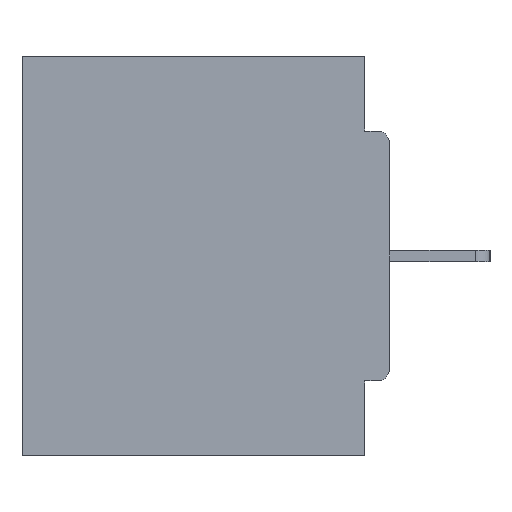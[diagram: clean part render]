
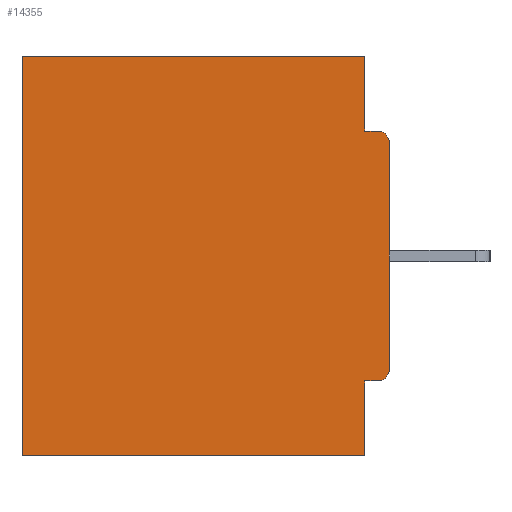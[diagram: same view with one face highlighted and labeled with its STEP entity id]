
A CAD part, left-side view. The second image highlights one B-rep face of the part: STEP entity #14355.
In plain terms, the highlighted planar face has unit normal (-1, 0, 0).
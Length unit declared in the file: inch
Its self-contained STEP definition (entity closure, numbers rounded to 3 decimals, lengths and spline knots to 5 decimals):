
#38 = CARTESIAN_POINT ( 'NONE',  ( 0.298, 0., -0.4065 ) ) ;
#102 = ORIENTED_EDGE ( 'NONE', *, *, #11221, .T. ) ;
#595 = DIRECTION ( 'NONE',  ( -1., 0., 0. ) ) ;
#1660 = LINE ( 'NONE', #21079, #13743 ) ;
#1907 = VERTEX_POINT ( 'NONE', #7659 ) ;
#2743 = CARTESIAN_POINT ( 'NONE',  ( 0.298, 0.015, -0.1085 ) ) ;
#3783 = ORIENTED_EDGE ( 'NONE', *, *, #19556, .F. ) ;
#4271 = EDGE_CURVE ( 'NONE', #1907, #17681, #12947, .T. ) ;
#4318 = CARTESIAN_POINT ( 'NONE',  ( 0.298, 0.031, -0.4065 ) ) ;
#4432 = ORIENTED_EDGE ( 'NONE', *, *, #5031, .F. ) ;
#4503 = DIRECTION ( 'NONE',  ( 1., 0., 0. ) ) ;
#4578 = EDGE_CURVE ( 'NONE', #23569, #7492, #11130, .T. ) ;
#4992 = DIRECTION ( 'NONE',  ( 0., 0., -1. ) ) ;
#5031 = EDGE_CURVE ( 'NONE', #18633, #25274, #25916, .T. ) ;
#5230 = DIRECTION ( 'NONE',  ( 0., 0., -1. ) ) ;
#5578 = VECTOR ( 'NONE', #26715, 39.37008 ) ;
#6106 = DIRECTION ( 'NONE',  ( 0., -1., 0. ) ) ;
#6432 = AXIS2_PLACEMENT_3D ( 'NONE', #2743, #595, #9349 ) ;
#6659 = CARTESIAN_POINT ( 'NONE',  ( 0.298, 0., 0. ) ) ;
#6816 = CARTESIAN_POINT ( 'NONE',  ( 0.298, 0.031, -0.5 ) ) ;
#7492 = VERTEX_POINT ( 'NONE', #19065 ) ;
#7659 = CARTESIAN_POINT ( 'NONE',  ( 0.298, 0.031, 0. ) ) ;
#7872 = CARTESIAN_POINT ( 'NONE',  ( 0.298, 0.015, -0.0935 ) ) ;
#8665 = VERTEX_POINT ( 'NONE', #9202 ) ;
#8872 = DIRECTION ( 'NONE',  ( -1., 0., 0. ) ) ;
#9202 = CARTESIAN_POINT ( 'NONE',  ( 0.298, 0., -0.3915 ) ) ;
#9349 = DIRECTION ( 'NONE',  ( 0., 0., -1. ) ) ;
#9413 = ORIENTED_EDGE ( 'NONE', *, *, #13356, .T. ) ;
#9640 = CIRCLE ( 'NONE', #6432, 0.015 ) ;
#10144 = ORIENTED_EDGE ( 'NONE', *, *, #26848, .T. ) ;
#10217 = LINE ( 'NONE', #12099, #11525 ) ;
#10304 = VECTOR ( 'NONE', #21458, 39.37008 ) ;
#10714 = ORIENTED_EDGE ( 'NONE', *, *, #10889, .F. ) ;
#10738 = ORIENTED_EDGE ( 'NONE', *, *, #12659, .F. ) ;
#10889 = EDGE_CURVE ( 'NONE', #17681, #24503, #1660, .T. ) ;
#11065 = CIRCLE ( 'NONE', #27132, 0.015 ) ;
#11130 = LINE ( 'NONE', #26096, #18118 ) ;
#11221 = EDGE_CURVE ( 'NONE', #17450, #7492, #14136, .T. ) ;
#11470 = CARTESIAN_POINT ( 'NONE',  ( 0.298, 0., -0.1085 ) ) ;
#11479 = CARTESIAN_POINT ( 'NONE',  ( 0.298, 0., 0. ) ) ;
#11525 = VECTOR ( 'NONE', #24638, 39.37008 ) ;
#11661 = EDGE_CURVE ( 'NONE', #12113, #24503, #9640, .T. ) ;
#12099 = CARTESIAN_POINT ( 'NONE',  ( 0.298, 0.031, -0.5 ) ) ;
#12113 = VERTEX_POINT ( 'NONE', #11470 ) ;
#12446 = AXIS2_PLACEMENT_3D ( 'NONE', #6659, #4503, #13289 ) ;
#12659 = EDGE_CURVE ( 'NONE', #25274, #23569, #10217, .T. ) ;
#12947 = LINE ( 'NONE', #19554, #15370 ) ;
#13289 = DIRECTION ( 'NONE',  ( 0., 0., -1. ) ) ;
#13356 = EDGE_CURVE ( 'NONE', #1907, #17450, #13492, .T. ) ;
#13492 = LINE ( 'NONE', #11479, #5578 ) ;
#13743 = VECTOR ( 'NONE', #6106, 39.37008 ) ;
#14115 = LINE ( 'NONE', #16570, #14943 ) ;
#14136 = LINE ( 'NONE', #20199, #18360 ) ;
#14355 = ADVANCED_FACE ( 'NONE', ( #17603 ), #24481, .F. ) ;
#14943 = VECTOR ( 'NONE', #23179, 39.37008 ) ;
#15370 = VECTOR ( 'NONE', #19130, 39.37008 ) ;
#16570 = CARTESIAN_POINT ( 'NONE',  ( 0.298, 0., 0. ) ) ;
#17450 = VERTEX_POINT ( 'NONE', #18506 ) ;
#17603 = FACE_OUTER_BOUND ( 'NONE', #24898, .T. ) ;
#17681 = VERTEX_POINT ( 'NONE', #23815 ) ;
#18078 = CARTESIAN_POINT ( 'NONE',  ( 0.298, 0.015, -0.3915 ) ) ;
#18118 = VECTOR ( 'NONE', #19628, 39.37008 ) ;
#18360 = VECTOR ( 'NONE', #5230, 39.37008 ) ;
#18506 = CARTESIAN_POINT ( 'NONE',  ( 0.298, 0.46, 0. ) ) ;
#18633 = VERTEX_POINT ( 'NONE', #22580 ) ;
#18969 = ORIENTED_EDGE ( 'NONE', *, *, #4271, .F. ) ;
#19065 = CARTESIAN_POINT ( 'NONE',  ( 0.298, 0.46, -0.5 ) ) ;
#19130 = DIRECTION ( 'NONE',  ( 0., 0., -1. ) ) ;
#19554 = CARTESIAN_POINT ( 'NONE',  ( 0.298, 0.031, -0.5 ) ) ;
#19556 = EDGE_CURVE ( 'NONE', #12113, #8665, #14115, .T. ) ;
#19628 = DIRECTION ( 'NONE',  ( 0., 1., 0. ) ) ;
#20199 = CARTESIAN_POINT ( 'NONE',  ( 0.298, 0.46, 0. ) ) ;
#21078 = ORIENTED_EDGE ( 'NONE', *, *, #4578, .F. ) ;
#21079 = CARTESIAN_POINT ( 'NONE',  ( 0.298, 0., -0.0935 ) ) ;
#21458 = DIRECTION ( 'NONE',  ( 0., 1., 0. ) ) ;
#22580 = CARTESIAN_POINT ( 'NONE',  ( 0.298, 0.015, -0.4065 ) ) ;
#23179 = DIRECTION ( 'NONE',  ( 0., 0., -1. ) ) ;
#23531 = ORIENTED_EDGE ( 'NONE', *, *, #11661, .T. ) ;
#23569 = VERTEX_POINT ( 'NONE', #6816 ) ;
#23815 = CARTESIAN_POINT ( 'NONE',  ( 0.298, 0.031, -0.0935 ) ) ;
#24481 = PLANE ( 'NONE',  #12446 ) ;
#24503 = VERTEX_POINT ( 'NONE', #7872 ) ;
#24638 = DIRECTION ( 'NONE',  ( 0., 0., -1. ) ) ;
#24898 = EDGE_LOOP ( 'NONE', ( #23531, #10714, #18969, #9413, #102, #21078, #10738, #4432, #10144, #3783 ) ) ;
#25274 = VERTEX_POINT ( 'NONE', #4318 ) ;
#25916 = LINE ( 'NONE', #38, #10304 ) ;
#26096 = CARTESIAN_POINT ( 'NONE',  ( 0.298, 0., -0.5 ) ) ;
#26715 = DIRECTION ( 'NONE',  ( 0., 1., 0. ) ) ;
#26848 = EDGE_CURVE ( 'NONE', #18633, #8665, #11065, .T. ) ;
#27132 = AXIS2_PLACEMENT_3D ( 'NONE', #18078, #8872, #4992 ) ;
